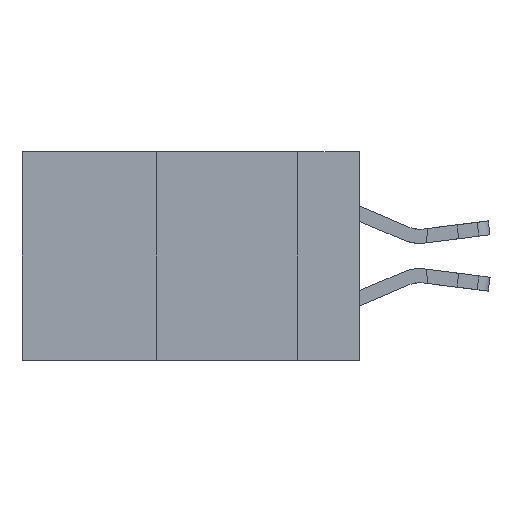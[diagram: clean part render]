
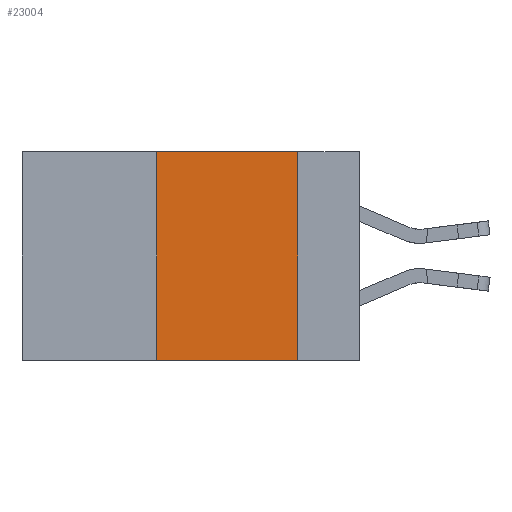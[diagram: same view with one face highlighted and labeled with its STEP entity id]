
A CAD part, left-side view. The second image highlights one B-rep face of the part: STEP entity #23004.
In plain terms, the highlighted planar face has unit normal (-1, 0, 0).
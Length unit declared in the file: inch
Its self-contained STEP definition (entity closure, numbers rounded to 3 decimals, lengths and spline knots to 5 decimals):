
#1138 = VECTOR ( 'NONE', #9962, 39.37008 ) ;
#1386 = PLANE ( 'NONE',  #21762 ) ;
#1713 = DIRECTION ( 'NONE',  ( 1., 0., 0. ) ) ;
#2866 = VECTOR ( 'NONE', #6159, 39.37008 ) ;
#3893 = CARTESIAN_POINT ( 'NONE',  ( 0., 0.36, -0.37 ) ) ;
#4098 = VERTEX_POINT ( 'NONE', #3893 ) ;
#4883 = EDGE_CURVE ( 'NONE', #5307, #21994, #19781, .T. ) ;
#4957 = CARTESIAN_POINT ( 'NONE',  ( 0., 0.11, 0. ) ) ;
#5307 = VERTEX_POINT ( 'NONE', #13612 ) ;
#6159 = DIRECTION ( 'NONE',  ( 0., -1., 0. ) ) ;
#6522 = CARTESIAN_POINT ( 'NONE',  ( 0., 0.6, -0.37 ) ) ;
#8355 = FACE_OUTER_BOUND ( 'NONE', #17474, .T. ) ;
#8574 = VECTOR ( 'NONE', #9910, 39.37008 ) ;
#9106 = LINE ( 'NONE', #25200, #2866 ) ;
#9910 = DIRECTION ( 'NONE',  ( 0., 0., 1. ) ) ;
#9962 = DIRECTION ( 'NONE',  ( 0., 0., -1. ) ) ;
#12696 = LINE ( 'NONE', #6522, #31703 ) ;
#13174 = ORIENTED_EDGE ( 'NONE', *, *, #13880, .T. ) ;
#13612 = CARTESIAN_POINT ( 'NONE',  ( 0., 0.11, 0. ) ) ;
#13805 = ORIENTED_EDGE ( 'NONE', *, *, #4883, .F. ) ;
#13880 = EDGE_CURVE ( 'NONE', #4098, #21994, #12696, .T. ) ;
#14127 = CARTESIAN_POINT ( 'NONE',  ( 0., 0.6, 0. ) ) ;
#14645 = ORIENTED_EDGE ( 'NONE', *, *, #15194, .F. ) ;
#15194 = EDGE_CURVE ( 'NONE', #31516, #5307, #9106, .T. ) ;
#17474 = EDGE_LOOP ( 'NONE', ( #13805, #14645, #31220, #13174 ) ) ;
#19781 = LINE ( 'NONE', #4957, #1138 ) ;
#21762 = AXIS2_PLACEMENT_3D ( 'NONE', #14127, #1713, #24157 ) ;
#21994 = VERTEX_POINT ( 'NONE', #26810 ) ;
#22045 = CARTESIAN_POINT ( 'NONE',  ( 0., 0.36, 0. ) ) ;
#23004 = ADVANCED_FACE ( 'NONE', ( #8355 ), #1386, .F. ) ;
#23815 = DIRECTION ( 'NONE',  ( 0., -1., 0. ) ) ;
#24157 = DIRECTION ( 'NONE',  ( 0., 0., -1. ) ) ;
#25200 = CARTESIAN_POINT ( 'NONE',  ( 0., 0.6, 0. ) ) ;
#25586 = LINE ( 'NONE', #22045, #8574 ) ;
#26810 = CARTESIAN_POINT ( 'NONE',  ( 0., 0.11, -0.37 ) ) ;
#29794 = EDGE_CURVE ( 'NONE', #4098, #31516, #25586, .T. ) ;
#31220 = ORIENTED_EDGE ( 'NONE', *, *, #29794, .F. ) ;
#31516 = VERTEX_POINT ( 'NONE', #32044 ) ;
#31703 = VECTOR ( 'NONE', #23815, 39.37008 ) ;
#32044 = CARTESIAN_POINT ( 'NONE',  ( 0., 0.36, 0. ) ) ;
